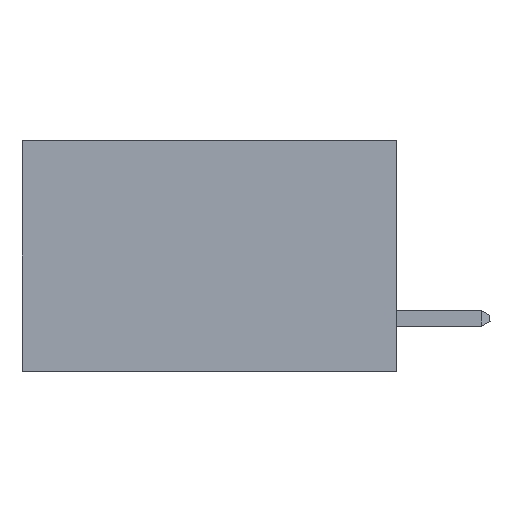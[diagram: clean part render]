
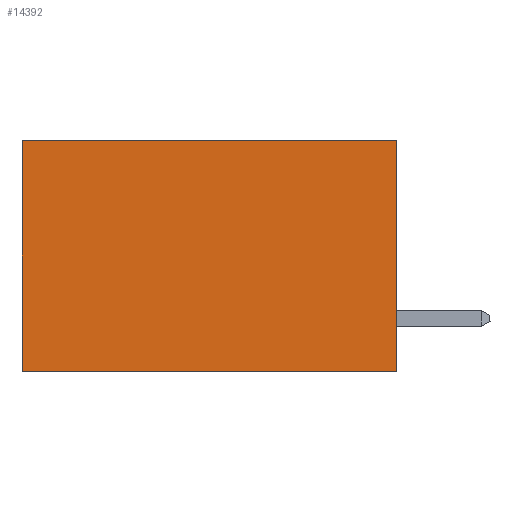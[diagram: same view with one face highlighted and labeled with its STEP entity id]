
A CAD part, left-side view. The second image highlights one B-rep face of the part: STEP entity #14392.
In plain terms, the highlighted planar face has unit normal (-1, 0, 0).
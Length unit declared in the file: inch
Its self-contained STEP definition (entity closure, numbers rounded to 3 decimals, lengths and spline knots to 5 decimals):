
#530 = LINE ( 'NONE', #2028, #15711 ) ;
#640 = CARTESIAN_POINT ( 'NONE',  ( 0.298, 0., 0. ) ) ;
#711 = VECTOR ( 'NONE', #14557, 39.37008 ) ;
#787 = FACE_OUTER_BOUND ( 'NONE', #8073, .T. ) ;
#1920 = DIRECTION ( 'NONE',  ( 1., 0., 0. ) ) ;
#2028 = CARTESIAN_POINT ( 'NONE',  ( 0.298, 0., -0.37 ) ) ;
#2162 = EDGE_CURVE ( 'NONE', #8206, #15345, #8416, .T. ) ;
#2209 = ORIENTED_EDGE ( 'NONE', *, *, #7674, .T. ) ;
#2577 = CARTESIAN_POINT ( 'NONE',  ( 0.298, 0., -0.37 ) ) ;
#3221 = EDGE_CURVE ( 'NONE', #8206, #17599, #19210, .T. ) ;
#3904 = DIRECTION ( 'NONE',  ( 0., 0., -1. ) ) ;
#4867 = CARTESIAN_POINT ( 'NONE',  ( 0.298, 0.6, 0. ) ) ;
#6332 = CARTESIAN_POINT ( 'NONE',  ( 0.298, 0., 0. ) ) ;
#6556 = DIRECTION ( 'NONE',  ( 0., 0., -1. ) ) ;
#7303 = AXIS2_PLACEMENT_3D ( 'NONE', #640, #1920, #6556 ) ;
#7674 = EDGE_CURVE ( 'NONE', #15345, #9714, #19852, .T. ) ;
#8073 = EDGE_LOOP ( 'NONE', ( #2209, #18791, #13068, #9015 ) ) ;
#8206 = VERTEX_POINT ( 'NONE', #6332 ) ;
#8416 = LINE ( 'NONE', #16338, #711 ) ;
#9015 = ORIENTED_EDGE ( 'NONE', *, *, #2162, .T. ) ;
#9714 = VERTEX_POINT ( 'NONE', #18500 ) ;
#9991 = VECTOR ( 'NONE', #11059, 39.37008 ) ;
#11059 = DIRECTION ( 'NONE',  ( 0., 0., -1. ) ) ;
#11077 = CARTESIAN_POINT ( 'NONE',  ( 0.298, 0.6, 0. ) ) ;
#13068 = ORIENTED_EDGE ( 'NONE', *, *, #3221, .F. ) ;
#14392 = ADVANCED_FACE ( 'NONE', ( #787 ), #15909, .F. ) ;
#14399 = DIRECTION ( 'NONE',  ( 0., 1., 0. ) ) ;
#14557 = DIRECTION ( 'NONE',  ( 0., 1., 0. ) ) ;
#15095 = VECTOR ( 'NONE', #3904, 39.37008 ) ;
#15345 = VERTEX_POINT ( 'NONE', #11077 ) ;
#15711 = VECTOR ( 'NONE', #14399, 39.37008 ) ;
#15909 = PLANE ( 'NONE',  #7303 ) ;
#16338 = CARTESIAN_POINT ( 'NONE',  ( 0.298, 0., 0. ) ) ;
#17173 = EDGE_CURVE ( 'NONE', #17599, #9714, #530, .T. ) ;
#17599 = VERTEX_POINT ( 'NONE', #2577 ) ;
#18500 = CARTESIAN_POINT ( 'NONE',  ( 0.298, 0.6, -0.37 ) ) ;
#18791 = ORIENTED_EDGE ( 'NONE', *, *, #17173, .F. ) ;
#19061 = CARTESIAN_POINT ( 'NONE',  ( 0.298, 0., 0. ) ) ;
#19210 = LINE ( 'NONE', #19061, #15095 ) ;
#19852 = LINE ( 'NONE', #4867, #9991 ) ;
